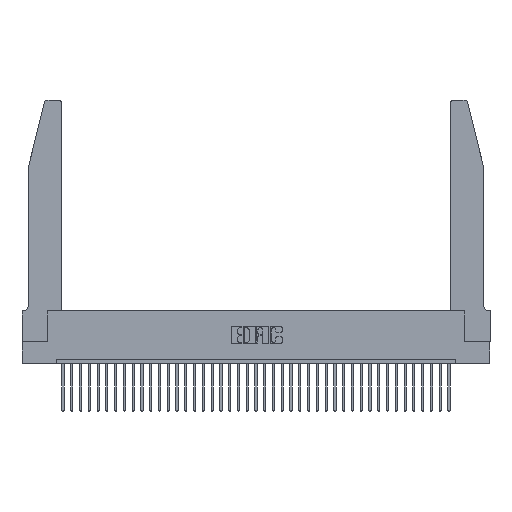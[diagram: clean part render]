
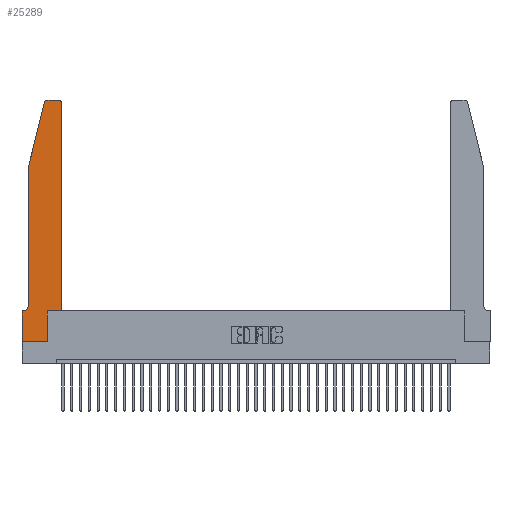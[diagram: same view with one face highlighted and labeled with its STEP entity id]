
A CAD part, top view. The second image highlights one B-rep face of the part: STEP entity #25289.
In plain terms, the highlighted planar face has unit normal (0, 0, 1).
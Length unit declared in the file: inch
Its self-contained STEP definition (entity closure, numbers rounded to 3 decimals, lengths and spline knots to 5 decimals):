
#334 = VERTEX_POINT ( 'NONE', #20978 ) ;
#621 = LINE ( 'NONE', #5251, #5292 ) ;
#2312 = EDGE_CURVE ( 'NONE', #20954, #2499, #32466, .T. ) ;
#2499 = VERTEX_POINT ( 'NONE', #23818 ) ;
#2869 = AXIS2_PLACEMENT_3D ( 'NONE', #19351, #28341, #22815 ) ;
#3879 = CARTESIAN_POINT ( 'NONE',  ( 0.0055, 0.42, 0.37 ) ) ;
#3974 = EDGE_CURVE ( 'NONE', #334, #34258, #27760, .T. ) ;
#4369 = DIRECTION ( 'NONE',  ( -1., 0., 0. ) ) ;
#5251 = CARTESIAN_POINT ( 'NONE',  ( 0., 0., 0.37 ) ) ;
#5282 = CARTESIAN_POINT ( 'NONE',  ( 0.4205, 2.72, 0.37 ) ) ;
#5292 = VECTOR ( 'NONE', #18515, 39.37008 ) ;
#5330 = DIRECTION ( 'NONE',  ( 1., 0., 0. ) ) ;
#6112 = ORIENTED_EDGE ( 'NONE', *, *, #12016, .T. ) ;
#6441 = CARTESIAN_POINT ( 'NONE',  ( 0.0755, 0.42, 0.37 ) ) ;
#6535 = VECTOR ( 'NONE', #32213, 39.37008 ) ;
#7242 = CARTESIAN_POINT ( 'NONE',  ( 0.0755, 0.35, 0.37 ) ) ;
#8140 = VERTEX_POINT ( 'NONE', #12853 ) ;
#8263 = CIRCLE ( 'NONE', #31992, 0.07 ) ;
#8434 = VERTEX_POINT ( 'NONE', #13158 ) ;
#8816 = DIRECTION ( 'NONE',  ( 0., 0., 1. ) ) ;
#9357 = AXIS2_PLACEMENT_3D ( 'NONE', #31917, #8816, #5330 ) ;
#9954 = DIRECTION ( 'NONE',  ( -1., 0., 0. ) ) ;
#9984 = CARTESIAN_POINT ( 'NONE',  ( 0.0055, 0.35, 0.37 ) ) ;
#10694 = EDGE_CURVE ( 'NONE', #34258, #22632, #33631, .T. ) ;
#10786 = CARTESIAN_POINT ( 'NONE',  ( 0.2605, 2.75, 0.37 ) ) ;
#11162 = ORIENTED_EDGE ( 'NONE', *, *, #23317, .T. ) ;
#11388 = AXIS2_PLACEMENT_3D ( 'NONE', #5282, #37762, #22980 ) ;
#11629 = FACE_OUTER_BOUND ( 'NONE', #19696, .T. ) ;
#11733 = DIRECTION ( 'NONE',  ( 1., 0., 0. ) ) ;
#12016 = EDGE_CURVE ( 'NONE', #18460, #8140, #16910, .T. ) ;
#12853 = CARTESIAN_POINT ( 'NONE',  ( 0.0755, 2., 0.37 ) ) ;
#13158 = CARTESIAN_POINT ( 'NONE',  ( 0.4205, 2.75, 0.37 ) ) ;
#13773 = VECTOR ( 'NONE', #13775, 39.37008 ) ;
#13775 = DIRECTION ( 'NONE',  ( -1., 0., 0. ) ) ;
#15431 = DIRECTION ( 'NONE',  ( 1., 0., 0. ) ) ;
#16097 = VECTOR ( 'NONE', #30777, 39.37008 ) ;
#16709 = LINE ( 'NONE', #26407, #6535 ) ;
#16910 = LINE ( 'NONE', #33981, #32570 ) ;
#17727 = CARTESIAN_POINT ( 'NONE',  ( 0.2865, 0., 0.37 ) ) ;
#18402 = CARTESIAN_POINT ( 'NONE',  ( 0., 0., 0.37 ) ) ;
#18460 = VERTEX_POINT ( 'NONE', #35595 ) ;
#18515 = DIRECTION ( 'NONE',  ( 0., -1., 0. ) ) ;
#19283 = VERTEX_POINT ( 'NONE', #17727 ) ;
#19351 = CARTESIAN_POINT ( 'NONE',  ( 0., 0.35, 0.37 ) ) ;
#19515 = VECTOR ( 'NONE', #15431, 39.37008 ) ;
#19696 = EDGE_LOOP ( 'NONE', ( #32306, #26562, #6112, #31504, #35216, #19961, #11162, #35042, #20492, #32152, #23746, #30315 ) ) ;
#19944 = VECTOR ( 'NONE', #11733, 39.37008 ) ;
#19961 = ORIENTED_EDGE ( 'NONE', *, *, #2312, .T. ) ;
#20110 = CIRCLE ( 'NONE', #11388, 0.03 ) ;
#20383 = VERTEX_POINT ( 'NONE', #30565 ) ;
#20492 = ORIENTED_EDGE ( 'NONE', *, *, #37426, .T. ) ;
#20771 = EDGE_CURVE ( 'NONE', #20383, #19283, #31487, .T. ) ;
#20954 = VERTEX_POINT ( 'NONE', #9984 ) ;
#20978 = CARTESIAN_POINT ( 'NONE',  ( 0.2865, 0.35, 0.37 ) ) ;
#21753 = CARTESIAN_POINT ( 'NONE',  ( 0.4505, 0.35, 0.37 ) ) ;
#22632 = VERTEX_POINT ( 'NONE', #36172 ) ;
#22815 = DIRECTION ( 'NONE',  ( 1., 0., 0. ) ) ;
#22980 = DIRECTION ( 'NONE',  ( 1., 0., 0. ) ) ;
#23317 = EDGE_CURVE ( 'NONE', #2499, #20383, #621, .T. ) ;
#23746 = ORIENTED_EDGE ( 'NONE', *, *, #10694, .T. ) ;
#23818 = CARTESIAN_POINT ( 'NONE',  ( 0., 0.35, 0.37 ) ) ;
#23948 = CARTESIAN_POINT ( 'NONE',  ( 0.4505, 0.35, 0.37 ) ) ;
#25016 = CIRCLE ( 'NONE', #9357, 0.03 ) ;
#25289 = ADVANCED_FACE ( 'NONE', ( #11629 ), #28604, .T. ) ;
#25577 = EDGE_CURVE ( 'NONE', #35902, #18460, #25016, .T. ) ;
#25745 = CARTESIAN_POINT ( 'NONE',  ( 0.2865, 0.35, 0.37 ) ) ;
#26407 = CARTESIAN_POINT ( 'NONE',  ( 0.0755, 2., 0.37 ) ) ;
#26562 = ORIENTED_EDGE ( 'NONE', *, *, #25577, .T. ) ;
#27393 = CARTESIAN_POINT ( 'NONE',  ( 0.284, 2.75, 0.37 ) ) ;
#27612 = DIRECTION ( 'NONE',  ( 0., 0., -1. ) ) ;
#27760 = LINE ( 'NONE', #37034, #19944 ) ;
#28341 = DIRECTION ( 'NONE',  ( 0., 0., 1. ) ) ;
#28604 = PLANE ( 'NONE',  #2869 ) ;
#28768 = VECTOR ( 'NONE', #4369, 39.37008 ) ;
#28788 = EDGE_CURVE ( 'NONE', #22632, #8434, #20110, .T. ) ;
#30315 = ORIENTED_EDGE ( 'NONE', *, *, #28788, .T. ) ;
#30385 = LINE ( 'NONE', #10786, #13773 ) ;
#30565 = CARTESIAN_POINT ( 'NONE',  ( 0., 0., 0.37 ) ) ;
#30777 = DIRECTION ( 'NONE',  ( 0., 1., 0. ) ) ;
#30941 = EDGE_CURVE ( 'NONE', #8140, #36437, #16709, .T. ) ;
#31487 = LINE ( 'NONE', #18402, #19515 ) ;
#31504 = ORIENTED_EDGE ( 'NONE', *, *, #30941, .T. ) ;
#31917 = CARTESIAN_POINT ( 'NONE',  ( 0.284, 2.72, 0.37 ) ) ;
#31992 = AXIS2_PLACEMENT_3D ( 'NONE', #3879, #27612, #9954 ) ;
#32152 = ORIENTED_EDGE ( 'NONE', *, *, #3974, .T. ) ;
#32213 = DIRECTION ( 'NONE',  ( 0., -1., 0. ) ) ;
#32306 = ORIENTED_EDGE ( 'NONE', *, *, #35532, .T. ) ;
#32466 = LINE ( 'NONE', #7242, #28768 ) ;
#32570 = VECTOR ( 'NONE', #34356, 39.37008 ) ;
#33218 = EDGE_CURVE ( 'NONE', #36437, #20954, #8263, .T. ) ;
#33631 = LINE ( 'NONE', #21753, #16097 ) ;
#33981 = CARTESIAN_POINT ( 'NONE',  ( 0.0755, 2., 0.37 ) ) ;
#34258 = VERTEX_POINT ( 'NONE', #23948 ) ;
#34334 = LINE ( 'NONE', #25745, #35694 ) ;
#34356 = DIRECTION ( 'NONE',  ( -0.239, -0.971, 0. ) ) ;
#35042 = ORIENTED_EDGE ( 'NONE', *, *, #20771, .T. ) ;
#35216 = ORIENTED_EDGE ( 'NONE', *, *, #33218, .T. ) ;
#35532 = EDGE_CURVE ( 'NONE', #8434, #35902, #30385, .T. ) ;
#35595 = CARTESIAN_POINT ( 'NONE',  ( 0.25487, 2.72718, 0.37 ) ) ;
#35694 = VECTOR ( 'NONE', #37573, 39.37008 ) ;
#35902 = VERTEX_POINT ( 'NONE', #27393 ) ;
#36172 = CARTESIAN_POINT ( 'NONE',  ( 0.4505, 2.72, 0.37 ) ) ;
#36437 = VERTEX_POINT ( 'NONE', #6441 ) ;
#37034 = CARTESIAN_POINT ( 'NONE',  ( 0.4505, 0.35, 0.37 ) ) ;
#37426 = EDGE_CURVE ( 'NONE', #19283, #334, #34334, .T. ) ;
#37573 = DIRECTION ( 'NONE',  ( 0., 1., 0. ) ) ;
#37762 = DIRECTION ( 'NONE',  ( 0., 0., 1. ) ) ;
